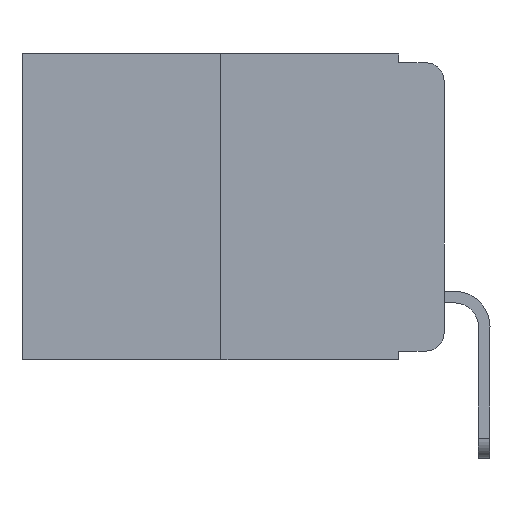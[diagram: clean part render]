
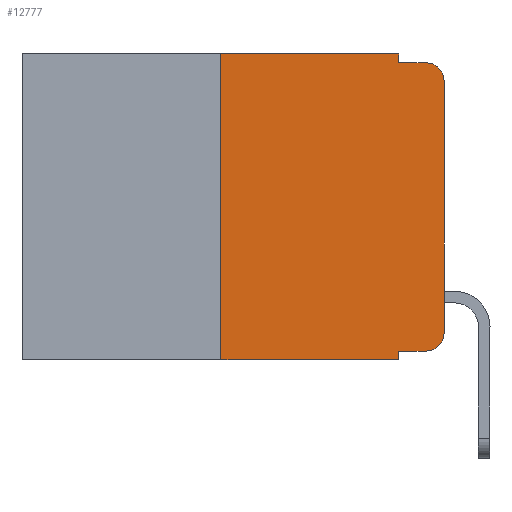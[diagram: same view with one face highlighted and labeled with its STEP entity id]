
A CAD part, left-side view. The second image highlights one B-rep face of the part: STEP entity #12777.
In plain terms, the highlighted planar face has unit normal (-1, 0, 0).
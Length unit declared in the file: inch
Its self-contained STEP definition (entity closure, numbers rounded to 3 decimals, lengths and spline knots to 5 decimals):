
#259 = DIRECTION ( 'NONE',  ( 0., 0., 1. ) ) ;
#499 = CARTESIAN_POINT ( 'NONE',  ( 0., 0.051, -0.343 ) ) ;
#528 = ORIENTED_EDGE ( 'NONE', *, *, #12106, .F. ) ;
#554 = VERTEX_POINT ( 'NONE', #6289 ) ;
#577 = LINE ( 'NONE', #3727, #5120 ) ;
#696 = DIRECTION ( 'NONE',  ( -1., 0., 0. ) ) ;
#758 = ORIENTED_EDGE ( 'NONE', *, *, #11588, .F. ) ;
#804 = VERTEX_POINT ( 'NONE', #5105 ) ;
#1010 = EDGE_CURVE ( 'NONE', #5238, #3771, #4350, .T. ) ;
#1147 = VECTOR ( 'NONE', #13313, 39.37008 ) ;
#1178 = VERTEX_POINT ( 'NONE', #7562 ) ;
#1768 = ORIENTED_EDGE ( 'NONE', *, *, #1010, .T. ) ;
#2774 = VECTOR ( 'NONE', #6890, 39.37008 ) ;
#2877 = DIRECTION ( 'NONE',  ( 0., 0., -1. ) ) ;
#3326 = EDGE_CURVE ( 'NONE', #15184, #4995, #14241, .T. ) ;
#3348 = VERTEX_POINT ( 'NONE', #5517 ) ;
#3587 = CARTESIAN_POINT ( 'NONE',  ( 0., 0.25, -0.343 ) ) ;
#3599 = ORIENTED_EDGE ( 'NONE', *, *, #3755, .F. ) ;
#3727 = CARTESIAN_POINT ( 'NONE',  ( 0., 0.051, 0. ) ) ;
#3755 = EDGE_CURVE ( 'NONE', #554, #4995, #11664, .T. ) ;
#3771 = VERTEX_POINT ( 'NONE', #6509 ) ;
#4107 = DIRECTION ( 'NONE',  ( 0., 0., -1. ) ) ;
#4133 = CARTESIAN_POINT ( 'NONE',  ( 0., 0., -0.03 ) ) ;
#4194 = AXIS2_PLACEMENT_3D ( 'NONE', #12208, #696, #4441 ) ;
#4350 = CIRCLE ( 'NONE', #11834, 0.02 ) ;
#4441 = DIRECTION ( 'NONE',  ( 0., 0., -1. ) ) ;
#4453 = AXIS2_PLACEMENT_3D ( 'NONE', #13826, #8958, #6237 ) ;
#4949 = ORIENTED_EDGE ( 'NONE', *, *, #5330, .T. ) ;
#4995 = VERTEX_POINT ( 'NONE', #499 ) ;
#5105 = CARTESIAN_POINT ( 'NONE',  ( 0., 0.25, 0. ) ) ;
#5120 = VECTOR ( 'NONE', #15034, 39.37008 ) ;
#5238 = VERTEX_POINT ( 'NONE', #8256 ) ;
#5330 = EDGE_CURVE ( 'NONE', #554, #5238, #10627, .T. ) ;
#5491 = DIRECTION ( 'NONE',  ( 0., -1., 0. ) ) ;
#5517 = CARTESIAN_POINT ( 'NONE',  ( 0., 0.051, -0.01 ) ) ;
#5706 = ORIENTED_EDGE ( 'NONE', *, *, #3326, .T. ) ;
#6123 = LINE ( 'NONE', #14562, #2774 ) ;
#6208 = ORIENTED_EDGE ( 'NONE', *, *, #7296, .T. ) ;
#6237 = DIRECTION ( 'NONE',  ( 0., 0., -1. ) ) ;
#6289 = CARTESIAN_POINT ( 'NONE',  ( 0., 0.051, -0.333 ) ) ;
#6509 = CARTESIAN_POINT ( 'NONE',  ( 0., 0., -0.313 ) ) ;
#6890 = DIRECTION ( 'NONE',  ( 0., 0., 1. ) ) ;
#7018 = CIRCLE ( 'NONE', #4194, 0.02 ) ;
#7296 = EDGE_CURVE ( 'NONE', #13732, #11504, #7018, .T. ) ;
#7373 = CARTESIAN_POINT ( 'NONE',  ( 0., 0.02, -0.01 ) ) ;
#7562 = CARTESIAN_POINT ( 'NONE',  ( 0., 0.051, 0. ) ) ;
#7711 = ORIENTED_EDGE ( 'NONE', *, *, #12238, .F. ) ;
#7735 = CARTESIAN_POINT ( 'NONE',  ( 0., 0.02, -0.313 ) ) ;
#7811 = CARTESIAN_POINT ( 'NONE',  ( 0., 0.25, 0. ) ) ;
#7849 = DIRECTION ( 'NONE',  ( -1., 0., 0. ) ) ;
#8021 = DIRECTION ( 'NONE',  ( 0., -1., 0. ) ) ;
#8256 = CARTESIAN_POINT ( 'NONE',  ( 0., 0.02, -0.333 ) ) ;
#8334 = VECTOR ( 'NONE', #4107, 39.37008 ) ;
#8909 = VECTOR ( 'NONE', #8021, 39.37008 ) ;
#8958 = DIRECTION ( 'NONE',  ( 1., 0., 0. ) ) ;
#9253 = LINE ( 'NONE', #11663, #13758 ) ;
#9461 = LINE ( 'NONE', #7811, #13769 ) ;
#9678 = VECTOR ( 'NONE', #5491, 39.37008 ) ;
#10410 = CARTESIAN_POINT ( 'NONE',  ( 0., 0.051, 0. ) ) ;
#10627 = LINE ( 'NONE', #13259, #1147 ) ;
#11002 = EDGE_CURVE ( 'NONE', #3348, #11504, #14787, .T. ) ;
#11175 = EDGE_CURVE ( 'NONE', #3771, #13732, #6123, .T. ) ;
#11295 = PLANE ( 'NONE',  #4453 ) ;
#11504 = VERTEX_POINT ( 'NONE', #7373 ) ;
#11588 = EDGE_CURVE ( 'NONE', #15184, #804, #9461, .T. ) ;
#11663 = CARTESIAN_POINT ( 'NONE',  ( 0., 0.473, 0. ) ) ;
#11664 = LINE ( 'NONE', #10410, #8334 ) ;
#11715 = EDGE_LOOP ( 'NONE', ( #15985, #6208, #16108, #528, #7711, #758, #5706, #3599, #4949, #1768 ) ) ;
#11834 = AXIS2_PLACEMENT_3D ( 'NONE', #7735, #7849, #2877 ) ;
#11909 = CARTESIAN_POINT ( 'NONE',  ( 0., 0.473, -0.343 ) ) ;
#12106 = EDGE_CURVE ( 'NONE', #1178, #3348, #577, .T. ) ;
#12208 = CARTESIAN_POINT ( 'NONE',  ( 0., 0.02, -0.03 ) ) ;
#12238 = EDGE_CURVE ( 'NONE', #804, #1178, #9253, .T. ) ;
#12777 = ADVANCED_FACE ( 'NONE', ( #15709 ), #11295, .F. ) ;
#13259 = CARTESIAN_POINT ( 'NONE',  ( 0., 0.051, -0.333 ) ) ;
#13313 = DIRECTION ( 'NONE',  ( 0., -1., 0. ) ) ;
#13732 = VERTEX_POINT ( 'NONE', #4133 ) ;
#13758 = VECTOR ( 'NONE', #15547, 39.37008 ) ;
#13769 = VECTOR ( 'NONE', #259, 39.37008 ) ;
#13826 = CARTESIAN_POINT ( 'NONE',  ( 0., 0.473, 0. ) ) ;
#14094 = CARTESIAN_POINT ( 'NONE',  ( 0., 0.051, -0.01 ) ) ;
#14241 = LINE ( 'NONE', #11909, #8909 ) ;
#14562 = CARTESIAN_POINT ( 'NONE',  ( 0., 0., 0. ) ) ;
#14787 = LINE ( 'NONE', #14094, #9678 ) ;
#15034 = DIRECTION ( 'NONE',  ( 0., 0., -1. ) ) ;
#15184 = VERTEX_POINT ( 'NONE', #3587 ) ;
#15547 = DIRECTION ( 'NONE',  ( 0., -1., 0. ) ) ;
#15709 = FACE_OUTER_BOUND ( 'NONE', #11715, .T. ) ;
#15985 = ORIENTED_EDGE ( 'NONE', *, *, #11175, .T. ) ;
#16108 = ORIENTED_EDGE ( 'NONE', *, *, #11002, .F. ) ;
